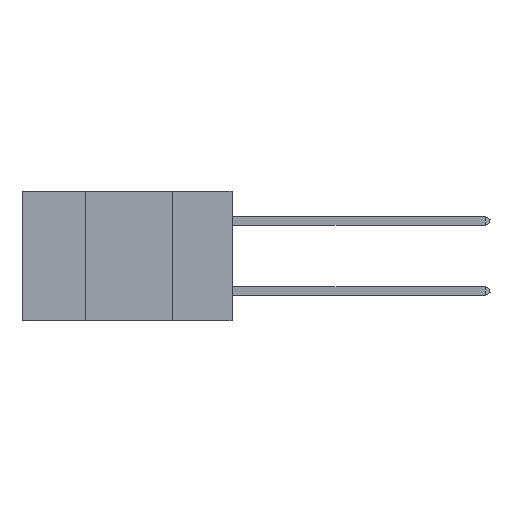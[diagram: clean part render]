
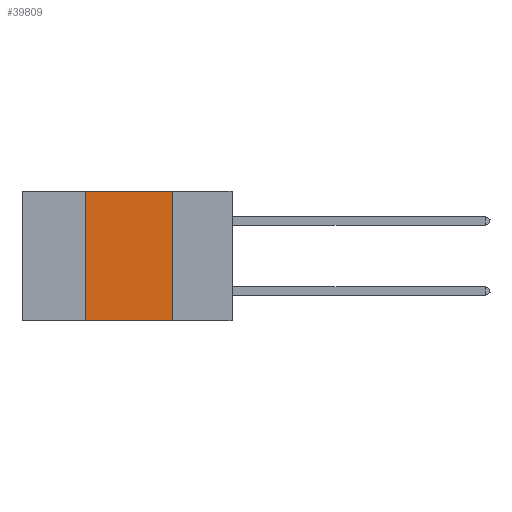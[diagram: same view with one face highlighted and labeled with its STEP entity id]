
A CAD part, left-side view. The second image highlights one B-rep face of the part: STEP entity #39809.
In plain terms, the highlighted planar face has unit normal (-1, 0, 0).
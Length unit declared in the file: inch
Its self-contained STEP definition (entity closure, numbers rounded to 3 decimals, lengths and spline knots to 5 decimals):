
#224 = VECTOR ( 'NONE', #41838, 39.37008 ) ;
#511 = VECTOR ( 'NONE', #35691, 39.37008 ) ;
#1341 = CARTESIAN_POINT ( 'NONE',  ( 0., 0.17, 0. ) ) ;
#2024 = CARTESIAN_POINT ( 'NONE',  ( 0., 0.17, -0.37 ) ) ;
#2145 = VERTEX_POINT ( 'NONE', #33293 ) ;
#3054 = LINE ( 'NONE', #13667, #17876 ) ;
#4551 = CARTESIAN_POINT ( 'NONE',  ( 0., 0.42, 0. ) ) ;
#4839 = EDGE_CURVE ( 'NONE', #2145, #6024, #19658, .T. ) ;
#6024 = VERTEX_POINT ( 'NONE', #2024 ) ;
#9911 = VERTEX_POINT ( 'NONE', #4551 ) ;
#10284 = LINE ( 'NONE', #31843, #224 ) ;
#12809 = CARTESIAN_POINT ( 'NONE',  ( 0., 0.42, -0.37 ) ) ;
#13667 = CARTESIAN_POINT ( 'NONE',  ( 0., 0.6, 0. ) ) ;
#13880 = ORIENTED_EDGE ( 'NONE', *, *, #4839, .F. ) ;
#15494 = DIRECTION ( 'NONE',  ( 0., -1., 0. ) ) ;
#15841 = DIRECTION ( 'NONE',  ( 1., 0., 0. ) ) ;
#16457 = LINE ( 'NONE', #25430, #24409 ) ;
#17212 = AXIS2_PLACEMENT_3D ( 'NONE', #19151, #15841, #42887 ) ;
#17876 = VECTOR ( 'NONE', #24183, 39.37008 ) ;
#18697 = VERTEX_POINT ( 'NONE', #12809 ) ;
#19060 = EDGE_CURVE ( 'NONE', #18697, #6024, #16457, .T. ) ;
#19151 = CARTESIAN_POINT ( 'NONE',  ( 0., 0.6, 0. ) ) ;
#19658 = LINE ( 'NONE', #1341, #511 ) ;
#24183 = DIRECTION ( 'NONE',  ( 0., -1., 0. ) ) ;
#24409 = VECTOR ( 'NONE', #15494, 39.37008 ) ;
#25430 = CARTESIAN_POINT ( 'NONE',  ( 0., 0.6, -0.37 ) ) ;
#30046 = ORIENTED_EDGE ( 'NONE', *, *, #19060, .T. ) ;
#31843 = CARTESIAN_POINT ( 'NONE',  ( 0., 0.42, 0. ) ) ;
#32167 = ORIENTED_EDGE ( 'NONE', *, *, #43963, .F. ) ;
#32467 = FACE_OUTER_BOUND ( 'NONE', #35924, .T. ) ;
#33293 = CARTESIAN_POINT ( 'NONE',  ( 0., 0.17, 0. ) ) ;
#35691 = DIRECTION ( 'NONE',  ( 0., 0., -1. ) ) ;
#35924 = EDGE_LOOP ( 'NONE', ( #13880, #32167, #42510, #30046 ) ) ;
#36316 = PLANE ( 'NONE',  #17212 ) ;
#37730 = EDGE_CURVE ( 'NONE', #18697, #9911, #10284, .T. ) ;
#39809 = ADVANCED_FACE ( 'NONE', ( #32467 ), #36316, .F. ) ;
#41838 = DIRECTION ( 'NONE',  ( 0., 0., 1. ) ) ;
#42510 = ORIENTED_EDGE ( 'NONE', *, *, #37730, .F. ) ;
#42887 = DIRECTION ( 'NONE',  ( 0., 0., -1. ) ) ;
#43963 = EDGE_CURVE ( 'NONE', #9911, #2145, #3054, .T. ) ;
